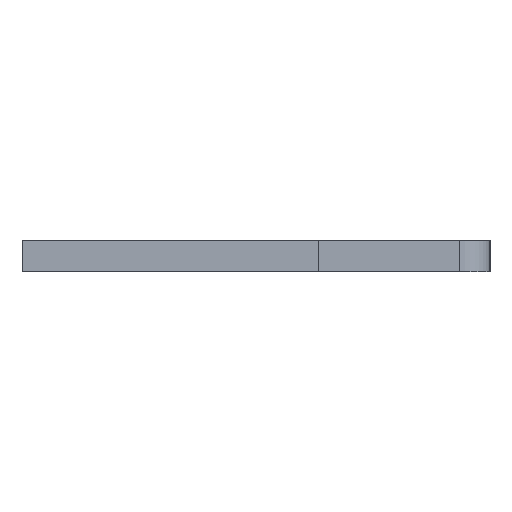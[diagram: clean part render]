
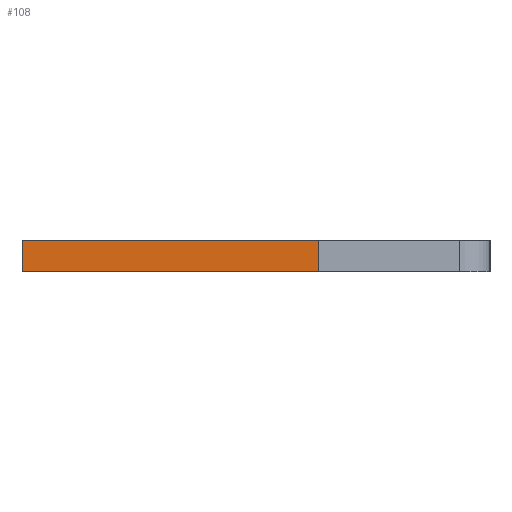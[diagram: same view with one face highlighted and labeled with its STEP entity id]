
A CAD part, left-side view. The second image highlights one B-rep face of the part: STEP entity #108.
In plain terms, the highlighted face is planar.
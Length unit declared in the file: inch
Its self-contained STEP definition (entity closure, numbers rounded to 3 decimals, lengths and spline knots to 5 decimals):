
#58 = LINE ( 'NONE', #1630, #141 ) ;
#76 = EDGE_CURVE ( 'NONE', #1535, #933, #2106, .T. ) ;
#108 = ADVANCED_FACE ( 'NONE', ( #621 ), #1769, .F. ) ;
#138 = ORIENTED_EDGE ( 'NONE', *, *, #1074, .T. ) ;
#141 = VECTOR ( 'NONE', #1801, 39.37008 ) ;
#144 = DIRECTION ( 'NONE',  ( 0., 1., 0. ) ) ;
#212 = VERTEX_POINT ( 'NONE', #1567 ) ;
#291 = ORIENTED_EDGE ( 'NONE', *, *, #76, .T. ) ;
#325 = DIRECTION ( 'NONE',  ( -1., 0., 0. ) ) ;
#502 = LINE ( 'NONE', #1137, #1049 ) ;
#548 = DIRECTION ( 'NONE',  ( -1., 0., 0. ) ) ;
#587 = CARTESIAN_POINT ( 'NONE',  ( 0.01, 0.15, -0.04 ) ) ;
#599 = VECTOR ( 'NONE', #325, 39.37008 ) ;
#621 = FACE_OUTER_BOUND ( 'NONE', #1007, .T. ) ;
#739 = ORIENTED_EDGE ( 'NONE', *, *, #1100, .F. ) ;
#821 = LINE ( 'NONE', #2018, #599 ) ;
#881 = CARTESIAN_POINT ( 'NONE',  ( 0.01, -0.04, -0.04 ) ) ;
#933 = VERTEX_POINT ( 'NONE', #1269 ) ;
#1007 = EDGE_LOOP ( 'NONE', ( #138, #1524, #739, #291 ) ) ;
#1036 = VECTOR ( 'NONE', #548, 39.37008 ) ;
#1049 = VECTOR ( 'NONE', #144, 39.37008 ) ;
#1074 = EDGE_CURVE ( 'NONE', #933, #212, #58, .T. ) ;
#1100 = EDGE_CURVE ( 'NONE', #1535, #1115, #502, .T. ) ;
#1115 = VERTEX_POINT ( 'NONE', #1978 ) ;
#1137 = CARTESIAN_POINT ( 'NONE',  ( 0.01, 0.15, -0.04 ) ) ;
#1146 = CARTESIAN_POINT ( 'NONE',  ( 0.01, -0.04, -0.04 ) ) ;
#1269 = CARTESIAN_POINT ( 'NONE',  ( -0.01, -0.04, -0.04 ) ) ;
#1414 = EDGE_CURVE ( 'NONE', #1115, #212, #821, .T. ) ;
#1432 = DIRECTION ( 'NONE',  ( 1., 0., 0. ) ) ;
#1481 = AXIS2_PLACEMENT_3D ( 'NONE', #587, #1774, #1432 ) ;
#1524 = ORIENTED_EDGE ( 'NONE', *, *, #1414, .F. ) ;
#1535 = VERTEX_POINT ( 'NONE', #1146 ) ;
#1567 = CARTESIAN_POINT ( 'NONE',  ( -0.01, 0.15, -0.04 ) ) ;
#1630 = CARTESIAN_POINT ( 'NONE',  ( -0.01, 0.15, -0.04 ) ) ;
#1769 = PLANE ( 'NONE',  #1481 ) ;
#1774 = DIRECTION ( 'NONE',  ( 0., 0., 1. ) ) ;
#1801 = DIRECTION ( 'NONE',  ( 0., 1., 0. ) ) ;
#1978 = CARTESIAN_POINT ( 'NONE',  ( 0.01, 0.15, -0.04 ) ) ;
#2018 = CARTESIAN_POINT ( 'NONE',  ( 0.01, 0.15, -0.04 ) ) ;
#2106 = LINE ( 'NONE', #881, #1036 ) ;
